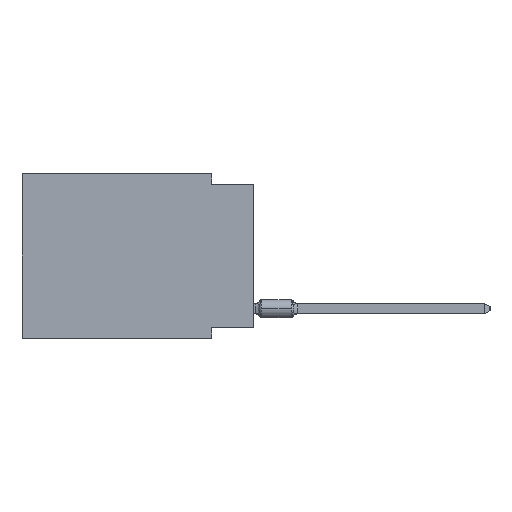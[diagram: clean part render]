
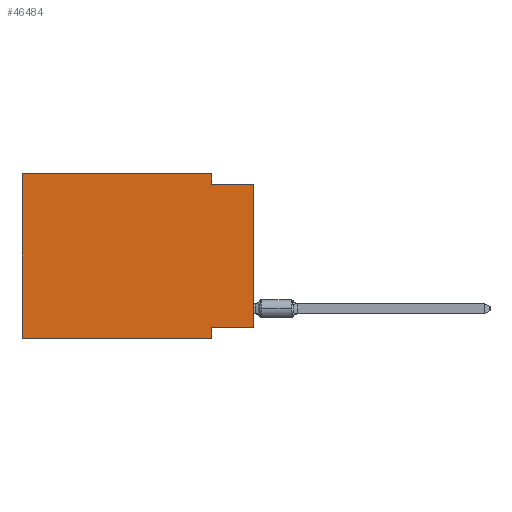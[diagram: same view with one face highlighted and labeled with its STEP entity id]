
A CAD part, left-side view. The second image highlights one B-rep face of the part: STEP entity #46484.
In plain terms, the highlighted planar face has unit normal (-1, 0, 0).
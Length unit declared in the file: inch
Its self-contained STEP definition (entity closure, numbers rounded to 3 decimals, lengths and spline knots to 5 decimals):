
#1560 = VECTOR ( 'NONE', #8052, 39.37008 ) ;
#2047 = EDGE_LOOP ( 'NONE', ( #14548, #6446, #14465, #50781, #38133, #50396, #9377, #19141 ) ) ;
#3362 = VERTEX_POINT ( 'NONE', #23861 ) ;
#4438 = LINE ( 'NONE', #46866, #38121 ) ;
#5605 = CARTESIAN_POINT ( 'NONE',  ( 0., 0.55, 0. ) ) ;
#6401 = CARTESIAN_POINT ( 'NONE',  ( 0., 0., -0.365 ) ) ;
#6446 = ORIENTED_EDGE ( 'NONE', *, *, #46807, .F. ) ;
#6686 = LINE ( 'NONE', #5605, #19640 ) ;
#7152 = DIRECTION ( 'NONE',  ( 0., -1., 0. ) ) ;
#8052 = DIRECTION ( 'NONE',  ( 0., 0., -1. ) ) ;
#9377 = ORIENTED_EDGE ( 'NONE', *, *, #28450, .F. ) ;
#9967 = LINE ( 'NONE', #35921, #20251 ) ;
#10071 = VERTEX_POINT ( 'NONE', #17788 ) ;
#10598 = DIRECTION ( 'NONE',  ( 0., -1., 0. ) ) ;
#10674 = CARTESIAN_POINT ( 'NONE',  ( 0., 0.55, -0.39 ) ) ;
#11055 = CARTESIAN_POINT ( 'NONE',  ( 0., 0., -0.025 ) ) ;
#11177 = PLANE ( 'NONE',  #16646 ) ;
#11376 = VECTOR ( 'NONE', #53217, 39.37008 ) ;
#11955 = EDGE_CURVE ( 'NONE', #35315, #16568, #6686, .T. ) ;
#14465 = ORIENTED_EDGE ( 'NONE', *, *, #31467, .F. ) ;
#14548 = ORIENTED_EDGE ( 'NONE', *, *, #29076, .T. ) ;
#14910 = CARTESIAN_POINT ( 'NONE',  ( 0., 0.1, 0. ) ) ;
#16568 = VERTEX_POINT ( 'NONE', #21771 ) ;
#16646 = AXIS2_PLACEMENT_3D ( 'NONE', #28220, #28500, #45269 ) ;
#17788 = CARTESIAN_POINT ( 'NONE',  ( 0., 0., -0.025 ) ) ;
#18077 = DIRECTION ( 'NONE',  ( 0., 0., 1. ) ) ;
#19141 = ORIENTED_EDGE ( 'NONE', *, *, #33084, .F. ) ;
#19640 = VECTOR ( 'NONE', #10598, 39.37008 ) ;
#20041 = LINE ( 'NONE', #54448, #1560 ) ;
#20251 = VECTOR ( 'NONE', #28084, 39.37008 ) ;
#21771 = CARTESIAN_POINT ( 'NONE',  ( 0., 0.1, 0. ) ) ;
#22144 = VECTOR ( 'NONE', #40616, 39.37008 ) ;
#23861 = CARTESIAN_POINT ( 'NONE',  ( 0., 0.1, -0.39 ) ) ;
#25023 = EDGE_CURVE ( 'NONE', #26721, #3362, #9967, .T. ) ;
#26125 = LINE ( 'NONE', #52945, #11376 ) ;
#26721 = VERTEX_POINT ( 'NONE', #10674 ) ;
#26869 = CARTESIAN_POINT ( 'NONE',  ( 0., 0.1, -0.365 ) ) ;
#28084 = DIRECTION ( 'NONE',  ( 0., -1., 0. ) ) ;
#28220 = CARTESIAN_POINT ( 'NONE',  ( 0., 0.55, 0. ) ) ;
#28229 = DIRECTION ( 'NONE',  ( 0., 1., 0. ) ) ;
#28450 = EDGE_CURVE ( 'NONE', #33005, #3362, #20041, .T. ) ;
#28500 = DIRECTION ( 'NONE',  ( 1., 0., 0. ) ) ;
#28648 = EDGE_CURVE ( 'NONE', #26721, #35315, #4438, .T. ) ;
#29076 = EDGE_CURVE ( 'NONE', #34510, #10071, #26125, .T. ) ;
#31467 = EDGE_CURVE ( 'NONE', #16568, #42243, #41179, .T. ) ;
#33005 = VERTEX_POINT ( 'NONE', #26869 ) ;
#33084 = EDGE_CURVE ( 'NONE', #34510, #33005, #45548, .T. ) ;
#34510 = VERTEX_POINT ( 'NONE', #6401 ) ;
#35315 = VERTEX_POINT ( 'NONE', #44240 ) ;
#35921 = CARTESIAN_POINT ( 'NONE',  ( 0., 0.55, -0.39 ) ) ;
#36630 = FACE_OUTER_BOUND ( 'NONE', #2047, .T. ) ;
#38121 = VECTOR ( 'NONE', #18077, 39.37008 ) ;
#38133 = ORIENTED_EDGE ( 'NONE', *, *, #28648, .F. ) ;
#40616 = DIRECTION ( 'NONE',  ( 0., 0., -1. ) ) ;
#41179 = LINE ( 'NONE', #14910, #22144 ) ;
#42243 = VERTEX_POINT ( 'NONE', #47575 ) ;
#42777 = VECTOR ( 'NONE', #28229, 39.37008 ) ;
#44240 = CARTESIAN_POINT ( 'NONE',  ( 0., 0.55, 0. ) ) ;
#45085 = VECTOR ( 'NONE', #7152, 39.37008 ) ;
#45269 = DIRECTION ( 'NONE',  ( 0., 0., -1. ) ) ;
#45548 = LINE ( 'NONE', #46094, #42777 ) ;
#46094 = CARTESIAN_POINT ( 'NONE',  ( 0., 0., -0.365 ) ) ;
#46484 = ADVANCED_FACE ( 'NONE', ( #36630 ), #11177, .F. ) ;
#46807 = EDGE_CURVE ( 'NONE', #42243, #10071, #54367, .T. ) ;
#46866 = CARTESIAN_POINT ( 'NONE',  ( 0., 0.55, 0. ) ) ;
#47575 = CARTESIAN_POINT ( 'NONE',  ( 0., 0.1, -0.025 ) ) ;
#50396 = ORIENTED_EDGE ( 'NONE', *, *, #25023, .T. ) ;
#50781 = ORIENTED_EDGE ( 'NONE', *, *, #11955, .F. ) ;
#52945 = CARTESIAN_POINT ( 'NONE',  ( 0., 0., 0. ) ) ;
#53217 = DIRECTION ( 'NONE',  ( 0., 0., 1. ) ) ;
#54367 = LINE ( 'NONE', #11055, #45085 ) ;
#54448 = CARTESIAN_POINT ( 'NONE',  ( 0., 0.1, -0.39 ) ) ;
